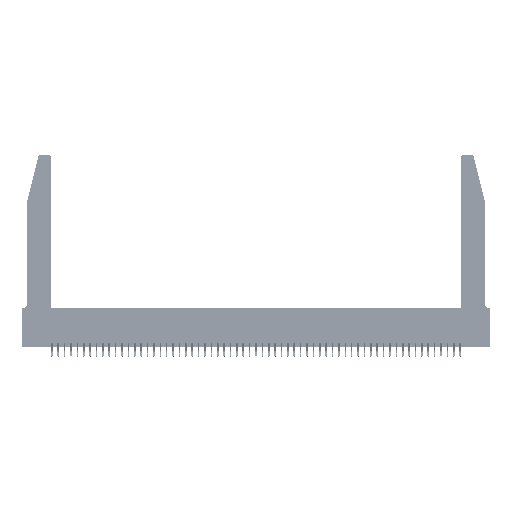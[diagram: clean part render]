
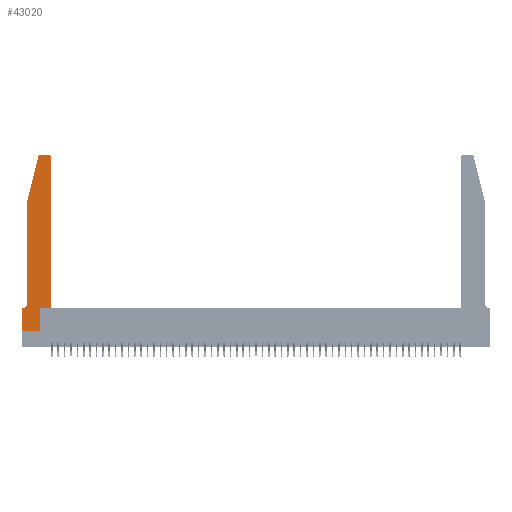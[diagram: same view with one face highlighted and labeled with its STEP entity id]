
A CAD part, top view. The second image highlights one B-rep face of the part: STEP entity #43020.
In plain terms, the highlighted planar face has unit normal (0, 0, 1).
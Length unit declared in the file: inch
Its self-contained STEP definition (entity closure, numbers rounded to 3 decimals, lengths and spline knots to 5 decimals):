
#111 = ORIENTED_EDGE ( 'NONE', *, *, #22077, .T. ) ;
#238 = CARTESIAN_POINT ( 'NONE',  ( 0.284, 2.72, 0.37 ) ) ;
#310 = EDGE_CURVE ( 'NONE', #52877, #9526, #19938, .T. ) ;
#3217 = VERTEX_POINT ( 'NONE', #27825 ) ;
#3321 = VECTOR ( 'NONE', #25024, 39.37008 ) ;
#3726 = PLANE ( 'NONE',  #47808 ) ;
#3851 = EDGE_CURVE ( 'NONE', #14656, #10805, #27291, .T. ) ;
#4080 = CARTESIAN_POINT ( 'NONE',  ( 0., 0.35, 0.37 ) ) ;
#4191 = ORIENTED_EDGE ( 'NONE', *, *, #10182, .T. ) ;
#4555 = CARTESIAN_POINT ( 'NONE',  ( 0.0755, 2., 0.37 ) ) ;
#4673 = ORIENTED_EDGE ( 'NONE', *, *, #310, .T. ) ;
#4838 = ORIENTED_EDGE ( 'NONE', *, *, #3851, .T. ) ;
#6615 = VERTEX_POINT ( 'NONE', #43267 ) ;
#7088 = DIRECTION ( 'NONE',  ( 0., 1., 0. ) ) ;
#7702 = EDGE_CURVE ( 'NONE', #27813, #42117, #27212, .T. ) ;
#7846 = DIRECTION ( 'NONE',  ( 0., 0., 1. ) ) ;
#8143 = CARTESIAN_POINT ( 'NONE',  ( 0.4505, 2.72, 0.37 ) ) ;
#8456 = DIRECTION ( 'NONE',  ( 0., 0., 1. ) ) ;
#8778 = DIRECTION ( 'NONE',  ( 1., 0., 0. ) ) ;
#9167 = EDGE_CURVE ( 'NONE', #43420, #17437, #17455, .T. ) ;
#9526 = VERTEX_POINT ( 'NONE', #43487 ) ;
#9973 = DIRECTION ( 'NONE',  ( 0., -1., 0. ) ) ;
#10182 = EDGE_CURVE ( 'NONE', #10805, #52877, #16679, .T. ) ;
#10535 = VECTOR ( 'NONE', #52459, 39.37008 ) ;
#10805 = VERTEX_POINT ( 'NONE', #31409 ) ;
#11395 = LINE ( 'NONE', #18722, #40222 ) ;
#13317 = ORIENTED_EDGE ( 'NONE', *, *, #7702, .T. ) ;
#13760 = ORIENTED_EDGE ( 'NONE', *, *, #50270, .T. ) ;
#14246 = AXIS2_PLACEMENT_3D ( 'NONE', #238, #8456, #28817 ) ;
#14595 = CARTESIAN_POINT ( 'NONE',  ( 0.0055, 0.35, 0.37 ) ) ;
#14625 = CARTESIAN_POINT ( 'NONE',  ( 0.0755, 0.35, 0.37 ) ) ;
#14656 = VERTEX_POINT ( 'NONE', #50418 ) ;
#15125 = DIRECTION ( 'NONE',  ( 1., 0., 0. ) ) ;
#15362 = LINE ( 'NONE', #4555, #17259 ) ;
#15764 = CARTESIAN_POINT ( 'NONE',  ( 0.0055, 0.42, 0.37 ) ) ;
#16609 = CARTESIAN_POINT ( 'NONE',  ( 0.2605, 2.75, 0.37 ) ) ;
#16679 = LINE ( 'NONE', #39814, #52495 ) ;
#17259 = VECTOR ( 'NONE', #29203, 39.37008 ) ;
#17437 = VERTEX_POINT ( 'NONE', #47713 ) ;
#17455 = CIRCLE ( 'NONE', #14246, 0.03 ) ;
#18722 = CARTESIAN_POINT ( 'NONE',  ( 0.0755, 2., 0.37 ) ) ;
#19168 = EDGE_CURVE ( 'NONE', #40409, #43420, #33356, .T. ) ;
#19938 = LINE ( 'NONE', #22840, #37866 ) ;
#20273 = LINE ( 'NONE', #46301, #44661 ) ;
#20521 = ORIENTED_EDGE ( 'NONE', *, *, #29177, .T. ) ;
#22077 = EDGE_CURVE ( 'NONE', #42117, #14656, #20273, .T. ) ;
#22289 = CARTESIAN_POINT ( 'NONE',  ( 0.284, 2.75, 0.37 ) ) ;
#22713 = ORIENTED_EDGE ( 'NONE', *, *, #41951, .T. ) ;
#22840 = CARTESIAN_POINT ( 'NONE',  ( 0.4505, 0.35, 0.37 ) ) ;
#24033 = AXIS2_PLACEMENT_3D ( 'NONE', #33608, #45663, #8778 ) ;
#25024 = DIRECTION ( 'NONE',  ( -1., 0., 0. ) ) ;
#26643 = DIRECTION ( 'NONE',  ( -1., 0., 0. ) ) ;
#27129 = DIRECTION ( 'NONE',  ( -1., 0., 0. ) ) ;
#27212 = LINE ( 'NONE', #14625, #36783 ) ;
#27291 = LINE ( 'NONE', #36432, #35583 ) ;
#27384 = ORIENTED_EDGE ( 'NONE', *, *, #46938, .T. ) ;
#27813 = VERTEX_POINT ( 'NONE', #14595 ) ;
#27825 = CARTESIAN_POINT ( 'NONE',  ( 0.0755, 2., 0.37 ) ) ;
#28196 = EDGE_LOOP ( 'NONE', ( #43567, #31201, #22713, #27384, #13760, #13317, #111, #4838, #4191, #4673, #20521, #29183 ) ) ;
#28765 = FACE_OUTER_BOUND ( 'NONE', #28196, .T. ) ;
#28769 = CARTESIAN_POINT ( 'NONE',  ( 0.4205, 2.75, 0.37 ) ) ;
#28817 = DIRECTION ( 'NONE',  ( 1., 0., 0. ) ) ;
#29177 = EDGE_CURVE ( 'NONE', #9526, #41822, #33609, .T. ) ;
#29183 = ORIENTED_EDGE ( 'NONE', *, *, #29999, .T. ) ;
#29203 = DIRECTION ( 'NONE',  ( -0.239, -0.971, 0. ) ) ;
#29999 = EDGE_CURVE ( 'NONE', #41822, #40409, #31571, .T. ) ;
#31201 = ORIENTED_EDGE ( 'NONE', *, *, #9167, .T. ) ;
#31409 = CARTESIAN_POINT ( 'NONE',  ( 0.2865, 0., 0.37 ) ) ;
#31571 = CIRCLE ( 'NONE', #24033, 0.03 ) ;
#32242 = DIRECTION ( 'NONE',  ( 0., 0., -1. ) ) ;
#32303 = AXIS2_PLACEMENT_3D ( 'NONE', #15764, #32242, #27129 ) ;
#33176 = CIRCLE ( 'NONE', #32303, 0.07 ) ;
#33356 = LINE ( 'NONE', #16609, #3321 ) ;
#33608 = CARTESIAN_POINT ( 'NONE',  ( 0.4205, 2.72, 0.37 ) ) ;
#33609 = LINE ( 'NONE', #39810, #10535 ) ;
#34380 = CARTESIAN_POINT ( 'NONE',  ( 0., 0.35, 0.37 ) ) ;
#35136 = DIRECTION ( 'NONE',  ( 0., -1., 0. ) ) ;
#35583 = VECTOR ( 'NONE', #40773, 39.37008 ) ;
#36415 = DIRECTION ( 'NONE',  ( 1., 0., 0. ) ) ;
#36432 = CARTESIAN_POINT ( 'NONE',  ( 0., 0., 0.37 ) ) ;
#36783 = VECTOR ( 'NONE', #26643, 39.37008 ) ;
#37866 = VECTOR ( 'NONE', #15125, 39.37008 ) ;
#39810 = CARTESIAN_POINT ( 'NONE',  ( 0.4505, 0.35, 0.37 ) ) ;
#39814 = CARTESIAN_POINT ( 'NONE',  ( 0.2865, 0.35, 0.37 ) ) ;
#40222 = VECTOR ( 'NONE', #35136, 39.37008 ) ;
#40409 = VERTEX_POINT ( 'NONE', #28769 ) ;
#40773 = DIRECTION ( 'NONE',  ( 1., 0., 0. ) ) ;
#41822 = VERTEX_POINT ( 'NONE', #8143 ) ;
#41951 = EDGE_CURVE ( 'NONE', #17437, #3217, #15362, .T. ) ;
#42117 = VERTEX_POINT ( 'NONE', #34380 ) ;
#43020 = ADVANCED_FACE ( 'NONE', ( #28765 ), #3726, .T. ) ;
#43267 = CARTESIAN_POINT ( 'NONE',  ( 0.0755, 0.42, 0.37 ) ) ;
#43420 = VERTEX_POINT ( 'NONE', #22289 ) ;
#43487 = CARTESIAN_POINT ( 'NONE',  ( 0.4505, 0.35, 0.37 ) ) ;
#43567 = ORIENTED_EDGE ( 'NONE', *, *, #19168, .T. ) ;
#44661 = VECTOR ( 'NONE', #9973, 39.37008 ) ;
#45663 = DIRECTION ( 'NONE',  ( 0., 0., 1. ) ) ;
#46301 = CARTESIAN_POINT ( 'NONE',  ( 0., 0., 0.37 ) ) ;
#46938 = EDGE_CURVE ( 'NONE', #3217, #6615, #11395, .T. ) ;
#47713 = CARTESIAN_POINT ( 'NONE',  ( 0.25487, 2.72718, 0.37 ) ) ;
#47808 = AXIS2_PLACEMENT_3D ( 'NONE', #4080, #7846, #36415 ) ;
#48286 = CARTESIAN_POINT ( 'NONE',  ( 0.2865, 0.35, 0.37 ) ) ;
#50270 = EDGE_CURVE ( 'NONE', #6615, #27813, #33176, .T. ) ;
#50418 = CARTESIAN_POINT ( 'NONE',  ( 0., 0., 0.37 ) ) ;
#52459 = DIRECTION ( 'NONE',  ( 0., 1., 0. ) ) ;
#52495 = VECTOR ( 'NONE', #7088, 39.37008 ) ;
#52877 = VERTEX_POINT ( 'NONE', #48286 ) ;
